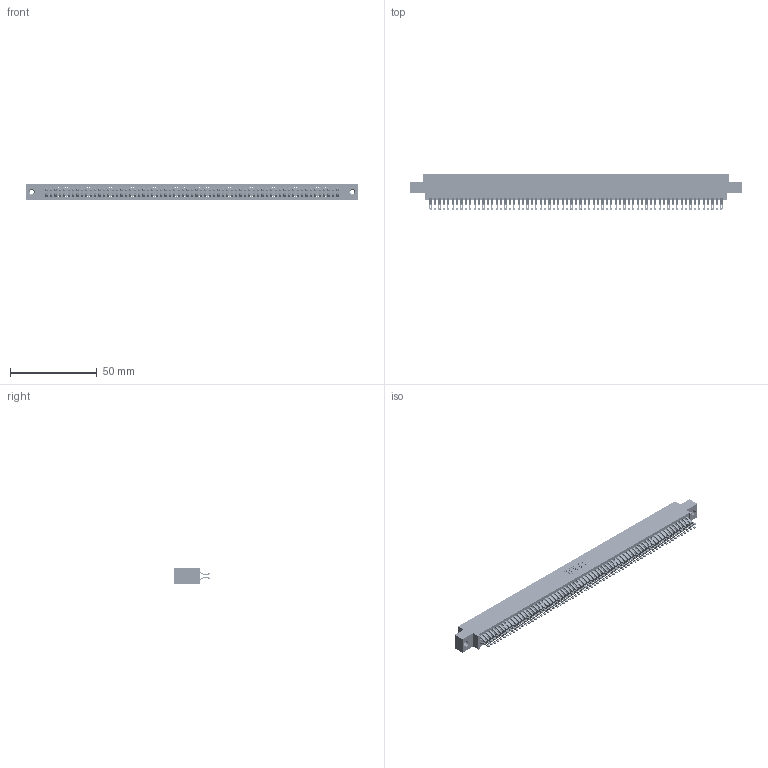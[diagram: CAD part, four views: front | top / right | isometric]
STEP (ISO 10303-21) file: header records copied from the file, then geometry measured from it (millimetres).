
FILE_DESCRIPTION (( 'STEP AP203' ), '1' );
FILE_NAME ('395-134-555-808.STEP', '2019-10-29T11:14:38', ( '' ), ( '' ), 'SwSTEP 2.0', 'SolidWorks 2016', '' );
FILE_SCHEMA (( 'CONFIG_CONTROL_DESIGN' ));
Length unit declared in the file: inch
Products named in the file (4): 395-134-555-808; 345 Part_0.170 Offset - 0.156 Dia-TI; 345-292-001_555 Tail; 345-250-001_345-250-003-102
Assembly tree (137 placements, depth 2):
  395-134-555-808
    345 Part_0.170 Offset - 0.156 Dia-TI
    345-292-001_555 Tail  x134
    345-250-001_345-250-003-102  x2
Bounding box: 191.39 x 21.13 x 9.4 mm (x, y, z)
Volume: 19092.6 mm3; surface area: 30214.9 mm2
Topology: 137 solids, 137 shells, 7694 faces, 24207 edges, 16130 vertices
Faces by surface type: plane 4270, cylinder 3408, cone 12, torus 4
Entity records: 50848 total; most frequent: CARTESIAN_POINT 8517, ORIENTED_EDGE 8414, DIRECTION 7473, EDGE_CURVE 4207, LINE 3767, VECTOR 3767, VERTEX_POINT 2800, AXIS2_PLACEMENT_3D 1853
